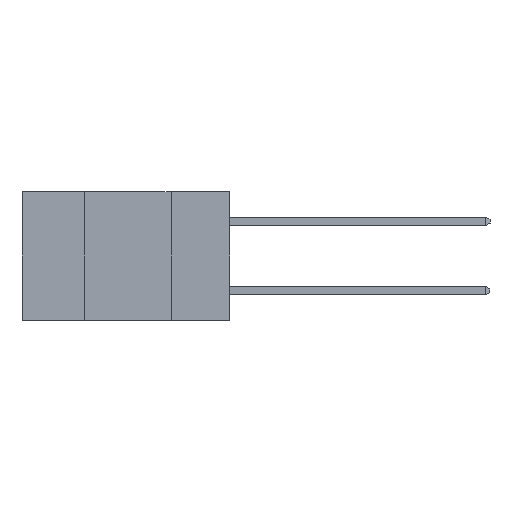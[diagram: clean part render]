
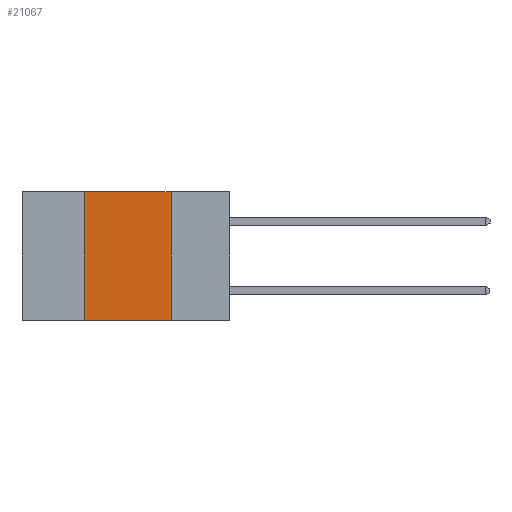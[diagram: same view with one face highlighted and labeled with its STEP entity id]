
A CAD part, left-side view. The second image highlights one B-rep face of the part: STEP entity #21067.
In plain terms, the highlighted planar face has unit normal (-1, 0, 0).
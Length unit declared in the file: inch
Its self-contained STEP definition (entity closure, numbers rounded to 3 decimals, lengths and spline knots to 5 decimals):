
#1413 = AXIS2_PLACEMENT_3D ( 'NONE', #12419, #3833, #15981 ) ;
#1567 = CARTESIAN_POINT ( 'NONE',  ( 0., 0.17, 0. ) ) ;
#1626 = VECTOR ( 'NONE', #9811, 39.37008 ) ;
#1666 = LINE ( 'NONE', #10442, #19504 ) ;
#3833 = DIRECTION ( 'NONE',  ( 1., 0., 0. ) ) ;
#5699 = CARTESIAN_POINT ( 'NONE',  ( 0., 0.17, -0.37 ) ) ;
#5838 = ORIENTED_EDGE ( 'NONE', *, *, #14345, .F. ) ;
#6145 = LINE ( 'NONE', #15018, #1626 ) ;
#6408 = VECTOR ( 'NONE', #22325, 39.37008 ) ;
#6911 = ORIENTED_EDGE ( 'NONE', *, *, #8734, .F. ) ;
#7510 = FACE_OUTER_BOUND ( 'NONE', #10949, .T. ) ;
#7890 = EDGE_CURVE ( 'NONE', #13077, #17782, #1666, .T. ) ;
#8734 = EDGE_CURVE ( 'NONE', #13077, #21068, #6145, .T. ) ;
#9448 = VERTEX_POINT ( 'NONE', #15905 ) ;
#9811 = DIRECTION ( 'NONE',  ( 0., 0., 1. ) ) ;
#10442 = CARTESIAN_POINT ( 'NONE',  ( 0., 0.6, -0.37 ) ) ;
#10568 = VECTOR ( 'NONE', #11775, 39.37008 ) ;
#10659 = PLANE ( 'NONE',  #1413 ) ;
#10949 = EDGE_LOOP ( 'NONE', ( #18069, #5838, #6911, #12007 ) ) ;
#11108 = LINE ( 'NONE', #22309, #10568 ) ;
#11775 = DIRECTION ( 'NONE',  ( 0., -1., 0. ) ) ;
#11906 = EDGE_CURVE ( 'NONE', #9448, #17782, #20262, .T. ) ;
#12007 = ORIENTED_EDGE ( 'NONE', *, *, #7890, .T. ) ;
#12419 = CARTESIAN_POINT ( 'NONE',  ( 0., 0.6, 0. ) ) ;
#13077 = VERTEX_POINT ( 'NONE', #17307 ) ;
#13983 = DIRECTION ( 'NONE',  ( 0., -1., 0. ) ) ;
#14345 = EDGE_CURVE ( 'NONE', #21068, #9448, #11108, .T. ) ;
#15018 = CARTESIAN_POINT ( 'NONE',  ( 0., 0.42, 0. ) ) ;
#15905 = CARTESIAN_POINT ( 'NONE',  ( 0., 0.17, 0. ) ) ;
#15906 = CARTESIAN_POINT ( 'NONE',  ( 0., 0.42, 0. ) ) ;
#15981 = DIRECTION ( 'NONE',  ( 0., 0., -1. ) ) ;
#17307 = CARTESIAN_POINT ( 'NONE',  ( 0., 0.42, -0.37 ) ) ;
#17782 = VERTEX_POINT ( 'NONE', #5699 ) ;
#18069 = ORIENTED_EDGE ( 'NONE', *, *, #11906, .F. ) ;
#19504 = VECTOR ( 'NONE', #13983, 39.37008 ) ;
#20262 = LINE ( 'NONE', #1567, #6408 ) ;
#21067 = ADVANCED_FACE ( 'NONE', ( #7510 ), #10659, .F. ) ;
#21068 = VERTEX_POINT ( 'NONE', #15906 ) ;
#22309 = CARTESIAN_POINT ( 'NONE',  ( 0., 0.6, 0. ) ) ;
#22325 = DIRECTION ( 'NONE',  ( 0., 0., -1. ) ) ;
